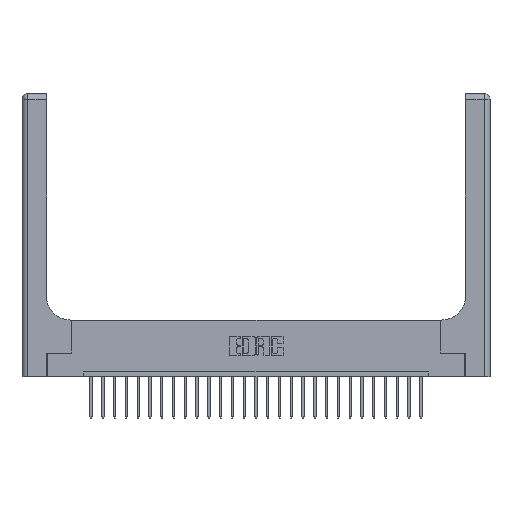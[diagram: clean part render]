
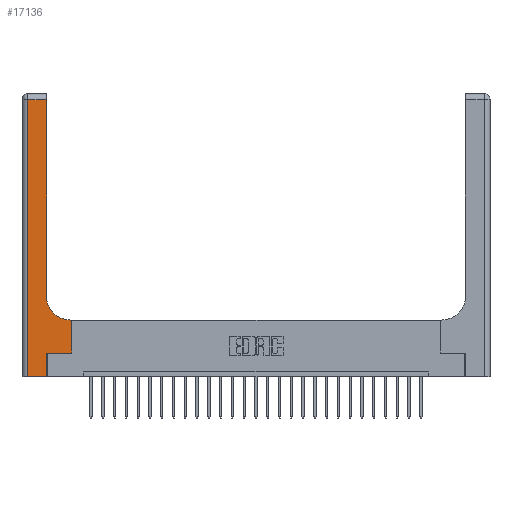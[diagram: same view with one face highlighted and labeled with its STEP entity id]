
A CAD part, top view. The second image highlights one B-rep face of the part: STEP entity #17136.
In plain terms, the highlighted planar face has unit normal (0, 0, 1).
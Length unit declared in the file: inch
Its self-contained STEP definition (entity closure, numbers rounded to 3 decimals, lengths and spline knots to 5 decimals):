
#202 = CARTESIAN_POINT ( 'NONE',  ( 0.265, 0.25, 0.37 ) ) ;
#484 = DIRECTION ( 'NONE',  ( 0., 1., 0. ) ) ;
#624 = DIRECTION ( 'NONE',  ( -1., 0., 0. ) ) ;
#665 = VERTEX_POINT ( 'NONE', #8665 ) ;
#1431 = EDGE_CURVE ( 'NONE', #12507, #19049, #4166, .T. ) ;
#2063 = VERTEX_POINT ( 'NONE', #14960 ) ;
#2698 = VECTOR ( 'NONE', #5008, 39.37008 ) ;
#3152 = FACE_OUTER_BOUND ( 'NONE', #11975, .T. ) ;
#3951 = ORIENTED_EDGE ( 'NONE', *, *, #21545, .T. ) ;
#4015 = LINE ( 'NONE', #15102, #20317 ) ;
#4166 = LINE ( 'NONE', #24020, #11108 ) ;
#4169 = LINE ( 'NONE', #6465, #13842 ) ;
#4184 = VERTEX_POINT ( 'NONE', #13984 ) ;
#4500 = PLANE ( 'NONE',  #11232 ) ;
#4888 = ORIENTED_EDGE ( 'NONE', *, *, #1431, .T. ) ;
#4901 = VECTOR ( 'NONE', #16616, 39.37008 ) ;
#5008 = DIRECTION ( 'NONE',  ( -1., 0., 0. ) ) ;
#5118 = ORIENTED_EDGE ( 'NONE', *, *, #14418, .T. ) ;
#5480 = LINE ( 'NONE', #23982, #24771 ) ;
#6274 = VECTOR ( 'NONE', #11693, 39.37008 ) ;
#6465 = CARTESIAN_POINT ( 'NONE',  ( 0.26, 3., 0.37 ) ) ;
#6504 = EDGE_CURVE ( 'NONE', #7609, #12507, #4015, .T. ) ;
#6639 = CARTESIAN_POINT ( 'NONE',  ( 0.51, 0.85, 0.37 ) ) ;
#7051 = CARTESIAN_POINT ( 'NONE',  ( 0.26, 0.6, 0.37 ) ) ;
#7422 = CARTESIAN_POINT ( 'NONE',  ( 0., 2.94, 0.37 ) ) ;
#7609 = VERTEX_POINT ( 'NONE', #14307 ) ;
#7811 = CARTESIAN_POINT ( 'NONE',  ( 0.528, 0.25, 0.37 ) ) ;
#8236 = CARTESIAN_POINT ( 'NONE',  ( 0., 3., 0.37 ) ) ;
#8441 = LINE ( 'NONE', #7051, #2698 ) ;
#8487 = EDGE_CURVE ( 'NONE', #4184, #665, #12074, .T. ) ;
#8519 = VERTEX_POINT ( 'NONE', #10766 ) ;
#8665 = CARTESIAN_POINT ( 'NONE',  ( 0.26, 0.85, 0.37 ) ) ;
#10766 = CARTESIAN_POINT ( 'NONE',  ( 0.528, 0.6, 0.37 ) ) ;
#11108 = VECTOR ( 'NONE', #18326, 39.37008 ) ;
#11232 = AXIS2_PLACEMENT_3D ( 'NONE', #8236, #20031, #624 ) ;
#11693 = DIRECTION ( 'NONE',  ( 0., 1., 0. ) ) ;
#11975 = EDGE_LOOP ( 'NONE', ( #5118, #24492, #23598, #4888, #15070, #18362, #20538, #3951, #14000 ) ) ;
#12074 = CIRCLE ( 'NONE', #19367, 0.25 ) ;
#12507 = VERTEX_POINT ( 'NONE', #13814 ) ;
#12703 = EDGE_CURVE ( 'NONE', #19049, #2063, #5480, .T. ) ;
#12959 = VECTOR ( 'NONE', #17288, 39.37008 ) ;
#13814 = CARTESIAN_POINT ( 'NONE',  ( 0.06, 0., 0.37 ) ) ;
#13842 = VECTOR ( 'NONE', #484, 39.37008 ) ;
#13974 = LINE ( 'NONE', #202, #4901 ) ;
#13984 = CARTESIAN_POINT ( 'NONE',  ( 0.51, 0.6, 0.37 ) ) ;
#14000 = ORIENTED_EDGE ( 'NONE', *, *, #8487, .T. ) ;
#14307 = CARTESIAN_POINT ( 'NONE',  ( 0.06, 2.94, 0.37 ) ) ;
#14418 = EDGE_CURVE ( 'NONE', #665, #18617, #4169, .T. ) ;
#14960 = CARTESIAN_POINT ( 'NONE',  ( 0.265, 0.25, 0.37 ) ) ;
#15070 = ORIENTED_EDGE ( 'NONE', *, *, #12703, .T. ) ;
#15102 = CARTESIAN_POINT ( 'NONE',  ( 0.06, 3., 0.37 ) ) ;
#15318 = CARTESIAN_POINT ( 'NONE',  ( 0.26, 2.94, 0.37 ) ) ;
#15337 = LINE ( 'NONE', #7811, #6274 ) ;
#15393 = EDGE_CURVE ( 'NONE', #17867, #8519, #15337, .T. ) ;
#15496 = CARTESIAN_POINT ( 'NONE',  ( 0.265, 0., 0.37 ) ) ;
#16154 = DIRECTION ( 'NONE',  ( 0., 1., 0. ) ) ;
#16616 = DIRECTION ( 'NONE',  ( 1., 0., 0. ) ) ;
#17026 = DIRECTION ( 'NONE',  ( 0., -1., 0. ) ) ;
#17136 = ADVANCED_FACE ( 'NONE', ( #3152 ), #4500, .F. ) ;
#17288 = DIRECTION ( 'NONE',  ( -1., 0., 0. ) ) ;
#17867 = VERTEX_POINT ( 'NONE', #19329 ) ;
#18094 = LINE ( 'NONE', #7422, #12959 ) ;
#18326 = DIRECTION ( 'NONE',  ( 1., 0., 0. ) ) ;
#18362 = ORIENTED_EDGE ( 'NONE', *, *, #20413, .T. ) ;
#18461 = DIRECTION ( 'NONE',  ( 0., 0., -1. ) ) ;
#18617 = VERTEX_POINT ( 'NONE', #15318 ) ;
#19049 = VERTEX_POINT ( 'NONE', #15496 ) ;
#19329 = CARTESIAN_POINT ( 'NONE',  ( 0.528, 0.25, 0.37 ) ) ;
#19367 = AXIS2_PLACEMENT_3D ( 'NONE', #6639, #18461, #20400 ) ;
#20031 = DIRECTION ( 'NONE',  ( 0., 0., -1. ) ) ;
#20317 = VECTOR ( 'NONE', #17026, 39.37008 ) ;
#20400 = DIRECTION ( 'NONE',  ( 1., 0., 0. ) ) ;
#20413 = EDGE_CURVE ( 'NONE', #2063, #17867, #13974, .T. ) ;
#20538 = ORIENTED_EDGE ( 'NONE', *, *, #15393, .T. ) ;
#21545 = EDGE_CURVE ( 'NONE', #8519, #4184, #8441, .T. ) ;
#22380 = EDGE_CURVE ( 'NONE', #18617, #7609, #18094, .T. ) ;
#23598 = ORIENTED_EDGE ( 'NONE', *, *, #6504, .T. ) ;
#23982 = CARTESIAN_POINT ( 'NONE',  ( 0.265, 0., 0.37 ) ) ;
#24020 = CARTESIAN_POINT ( 'NONE',  ( 0., 0., 0.37 ) ) ;
#24492 = ORIENTED_EDGE ( 'NONE', *, *, #22380, .T. ) ;
#24771 = VECTOR ( 'NONE', #16154, 39.37008 ) ;
